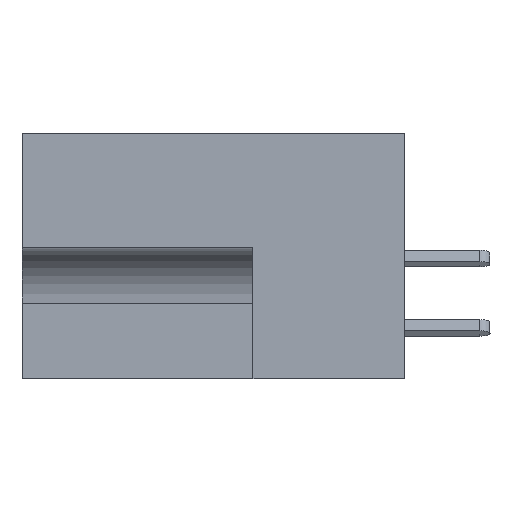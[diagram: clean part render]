
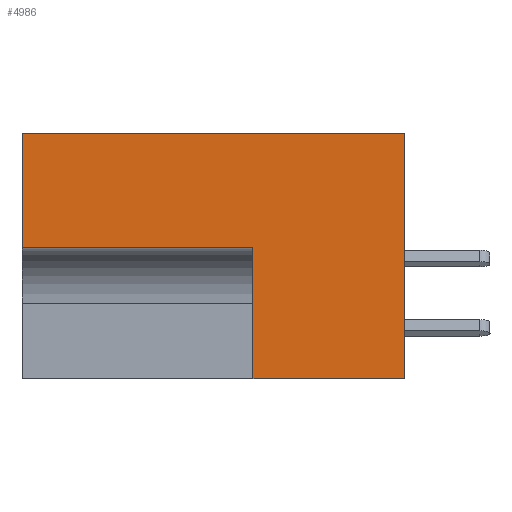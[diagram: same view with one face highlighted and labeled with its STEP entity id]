
A CAD part, left-side view. The second image highlights one B-rep face of the part: STEP entity #4986.
In plain terms, the highlighted planar face has unit normal (-1, 0, 0).
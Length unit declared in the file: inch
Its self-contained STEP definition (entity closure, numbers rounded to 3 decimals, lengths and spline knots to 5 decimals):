
#829 = CARTESIAN_POINT ( 'NONE',  ( 0., 0.328, -0.248 ) ) ;
#931 = LINE ( 'NONE', #3535, #5187 ) ;
#1119 = DIRECTION ( 'NONE',  ( 0., -1., 0. ) ) ;
#2159 = LINE ( 'NONE', #829, #15177 ) ;
#3535 = CARTESIAN_POINT ( 'NONE',  ( 0., 0.453, 0. ) ) ;
#3547 = CARTESIAN_POINT ( 'NONE',  ( 0., 0.453, -0.531 ) ) ;
#4522 = FACE_OUTER_BOUND ( 'NONE', #5977, .T. ) ;
#4986 = ADVANCED_FACE ( 'NONE', ( #4522 ), #29132, .F. ) ;
#5187 = VECTOR ( 'NONE', #1119, 39.37008 ) ;
#5628 = ORIENTED_EDGE ( 'NONE', *, *, #31539, .F. ) ;
#5977 = EDGE_LOOP ( 'NONE', ( #5628, #18684, #20542, #19204, #30907, #24310 ) ) ;
#6534 = VERTEX_POINT ( 'NONE', #14679 ) ;
#9649 = CARTESIAN_POINT ( 'NONE',  ( 0., 0., 0. ) ) ;
#9857 = EDGE_CURVE ( 'NONE', #26311, #12800, #15162, .T. ) ;
#11508 = CARTESIAN_POINT ( 'NONE',  ( 0., 0.328, -0.248 ) ) ;
#11750 = VERTEX_POINT ( 'NONE', #31559 ) ;
#12800 = VERTEX_POINT ( 'NONE', #9649 ) ;
#12845 = LINE ( 'NONE', #16658, #17123 ) ;
#13793 = EDGE_CURVE ( 'NONE', #25948, #11750, #2159, .T. ) ;
#14294 = CARTESIAN_POINT ( 'NONE',  ( 0., 0., -0.531 ) ) ;
#14387 = DIRECTION ( 'NONE',  ( 0., 0., -1. ) ) ;
#14679 = CARTESIAN_POINT ( 'NONE',  ( 0., 0.328, -0.531 ) ) ;
#15162 = LINE ( 'NONE', #26343, #25555 ) ;
#15177 = VECTOR ( 'NONE', #24995, 39.37008 ) ;
#15279 = CARTESIAN_POINT ( 'NONE',  ( 0., 0.828, 0. ) ) ;
#15710 = AXIS2_PLACEMENT_3D ( 'NONE', #31613, #16806, #14387 ) ;
#16350 = VECTOR ( 'NONE', #19575, 39.37008 ) ;
#16658 = CARTESIAN_POINT ( 'NONE',  ( 0., 0.328, -0.531 ) ) ;
#16806 = DIRECTION ( 'NONE',  ( 1., 0., 0. ) ) ;
#17123 = VECTOR ( 'NONE', #21583, 39.37008 ) ;
#18684 = ORIENTED_EDGE ( 'NONE', *, *, #13793, .F. ) ;
#18919 = EDGE_CURVE ( 'NONE', #6534, #26311, #31414, .T. ) ;
#19204 = ORIENTED_EDGE ( 'NONE', *, *, #18919, .T. ) ;
#19575 = DIRECTION ( 'NONE',  ( 0., 0., 1. ) ) ;
#20242 = VECTOR ( 'NONE', #30550, 39.37008 ) ;
#20542 = ORIENTED_EDGE ( 'NONE', *, *, #25723, .F. ) ;
#21583 = DIRECTION ( 'NONE',  ( 0., 0., 1. ) ) ;
#21703 = DIRECTION ( 'NONE',  ( 0., 0., 1. ) ) ;
#24310 = ORIENTED_EDGE ( 'NONE', *, *, #26598, .F. ) ;
#24995 = DIRECTION ( 'NONE',  ( 0., 1., 0. ) ) ;
#25555 = VECTOR ( 'NONE', #21703, 39.37008 ) ;
#25723 = EDGE_CURVE ( 'NONE', #6534, #25948, #12845, .T. ) ;
#25948 = VERTEX_POINT ( 'NONE', #11508 ) ;
#26311 = VERTEX_POINT ( 'NONE', #14294 ) ;
#26343 = CARTESIAN_POINT ( 'NONE',  ( 0., 0., 0. ) ) ;
#26598 = EDGE_CURVE ( 'NONE', #29697, #12800, #931, .T. ) ;
#29132 = PLANE ( 'NONE',  #15710 ) ;
#29356 = CARTESIAN_POINT ( 'NONE',  ( 0., 0.828, 0. ) ) ;
#29697 = VERTEX_POINT ( 'NONE', #15279 ) ;
#30202 = LINE ( 'NONE', #29356, #16350 ) ;
#30550 = DIRECTION ( 'NONE',  ( 0., -1., 0. ) ) ;
#30907 = ORIENTED_EDGE ( 'NONE', *, *, #9857, .T. ) ;
#31414 = LINE ( 'NONE', #3547, #20242 ) ;
#31539 = EDGE_CURVE ( 'NONE', #11750, #29697, #30202, .T. ) ;
#31559 = CARTESIAN_POINT ( 'NONE',  ( 0., 0.828, -0.248 ) ) ;
#31613 = CARTESIAN_POINT ( 'NONE',  ( 0., 0.453, 0. ) ) ;
